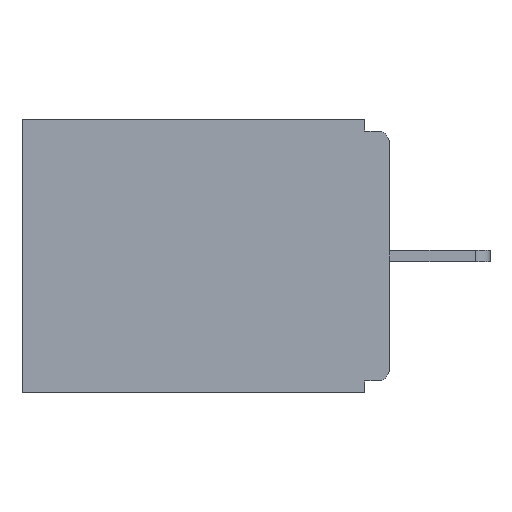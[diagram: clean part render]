
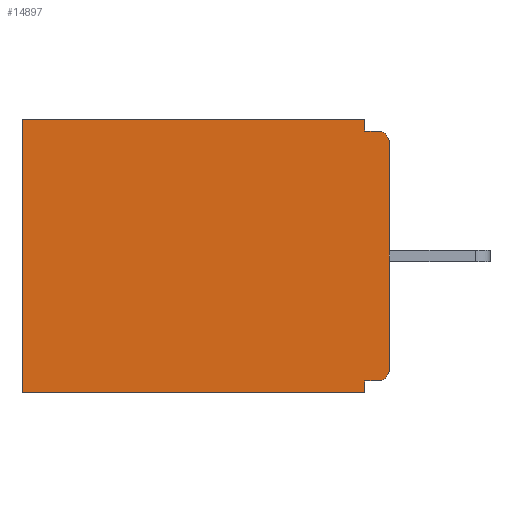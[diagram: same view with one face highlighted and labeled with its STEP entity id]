
A CAD part, left-side view. The second image highlights one B-rep face of the part: STEP entity #14897.
In plain terms, the highlighted planar face has unit normal (-1, 0, 0).
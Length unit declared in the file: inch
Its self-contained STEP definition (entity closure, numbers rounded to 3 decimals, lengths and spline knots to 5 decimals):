
#265 = EDGE_CURVE ( 'NONE', #14477, #7572, #15498, .T. ) ;
#371 = EDGE_CURVE ( 'NONE', #390, #12524, #1767, .T. ) ;
#390 = VERTEX_POINT ( 'NONE', #3162 ) ;
#401 = DIRECTION ( 'NONE',  ( 0., 1., 0. ) ) ;
#424 = CARTESIAN_POINT ( 'NONE',  ( 0.298, 0.031, -0.343 ) ) ;
#510 = DIRECTION ( 'NONE',  ( 0., 0., -1. ) ) ;
#1000 = ORIENTED_EDGE ( 'NONE', *, *, #10080, .T. ) ;
#1249 = VERTEX_POINT ( 'NONE', #15318 ) ;
#1595 = CARTESIAN_POINT ( 'NONE',  ( 0.298, 0.015, -0.015 ) ) ;
#1767 = CIRCLE ( 'NONE', #13955, 0.015 ) ;
#1855 = ORIENTED_EDGE ( 'NONE', *, *, #13545, .T. ) ;
#1878 = DIRECTION ( 'NONE',  ( -1., 0., 0. ) ) ;
#1902 = CARTESIAN_POINT ( 'NONE',  ( 0.298, 0.015, -0.313 ) ) ;
#2072 = DIRECTION ( 'NONE',  ( 0., -1., 0. ) ) ;
#2121 = EDGE_CURVE ( 'NONE', #4747, #12524, #15303, .T. ) ;
#2176 = CARTESIAN_POINT ( 'NONE',  ( 0.298, 0., -0.343 ) ) ;
#2389 = PLANE ( 'NONE',  #13708 ) ;
#2794 = DIRECTION ( 'NONE',  ( 0., 0., -1. ) ) ;
#2923 = FACE_OUTER_BOUND ( 'NONE', #7731, .T. ) ;
#3092 = EDGE_CURVE ( 'NONE', #7572, #6786, #9035, .T. ) ;
#3162 = CARTESIAN_POINT ( 'NONE',  ( 0.298, 0.015, -0.328 ) ) ;
#3292 = DIRECTION ( 'NONE',  ( 0., 0., -1. ) ) ;
#3473 = LINE ( 'NONE', #13514, #15269 ) ;
#3671 = DIRECTION ( 'NONE',  ( 0., 0., -1. ) ) ;
#4025 = ORIENTED_EDGE ( 'NONE', *, *, #11641, .F. ) ;
#4433 = ORIENTED_EDGE ( 'NONE', *, *, #13914, .T. ) ;
#4747 = VERTEX_POINT ( 'NONE', #12264 ) ;
#4798 = ORIENTED_EDGE ( 'NONE', *, *, #265, .F. ) ;
#5323 = VECTOR ( 'NONE', #15557, 39.37008 ) ;
#5744 = CIRCLE ( 'NONE', #6519, 0.015 ) ;
#5951 = VERTEX_POINT ( 'NONE', #9161 ) ;
#6136 = CARTESIAN_POINT ( 'NONE',  ( 0.298, 0., 0. ) ) ;
#6239 = VERTEX_POINT ( 'NONE', #12287 ) ;
#6481 = LINE ( 'NONE', #13273, #7225 ) ;
#6489 = CARTESIAN_POINT ( 'NONE',  ( 0.298, 0.031, 0. ) ) ;
#6519 = AXIS2_PLACEMENT_3D ( 'NONE', #13841, #6824, #14924 ) ;
#6579 = EDGE_CURVE ( 'NONE', #390, #1249, #6481, .T. ) ;
#6786 = VERTEX_POINT ( 'NONE', #1595 ) ;
#6824 = DIRECTION ( 'NONE',  ( -1., 0., 0. ) ) ;
#7225 = VECTOR ( 'NONE', #8311, 39.37008 ) ;
#7572 = VERTEX_POINT ( 'NONE', #7694 ) ;
#7694 = CARTESIAN_POINT ( 'NONE',  ( 0.298, 0.031, -0.015 ) ) ;
#7731 = EDGE_LOOP ( 'NONE', ( #1855, #13896, #4798, #1000, #4433, #10118, #4025, #14585, #8482, #14934 ) ) ;
#7816 = EDGE_CURVE ( 'NONE', #10622, #6239, #14106, .T. ) ;
#7980 = VECTOR ( 'NONE', #9443, 39.37008 ) ;
#8311 = DIRECTION ( 'NONE',  ( 0., 1., 0. ) ) ;
#8482 = ORIENTED_EDGE ( 'NONE', *, *, #371, .T. ) ;
#8664 = VECTOR ( 'NONE', #2072, 39.37008 ) ;
#8767 = CARTESIAN_POINT ( 'NONE',  ( 0.298, 0.46, 0. ) ) ;
#8950 = LINE ( 'NONE', #8767, #5323 ) ;
#9035 = LINE ( 'NONE', #9252, #8664 ) ;
#9161 = CARTESIAN_POINT ( 'NONE',  ( 0.298, 0.46, 0. ) ) ;
#9252 = CARTESIAN_POINT ( 'NONE',  ( 0.298, 0., -0.015 ) ) ;
#9385 = LINE ( 'NONE', #11911, #15061 ) ;
#9443 = DIRECTION ( 'NONE',  ( 0., 1., 0. ) ) ;
#10066 = CARTESIAN_POINT ( 'NONE',  ( 0.298, 0., -0.313 ) ) ;
#10080 = EDGE_CURVE ( 'NONE', #14477, #5951, #3473, .T. ) ;
#10118 = ORIENTED_EDGE ( 'NONE', *, *, #7816, .F. ) ;
#10256 = CARTESIAN_POINT ( 'NONE',  ( 0.298, 0., 0. ) ) ;
#10583 = VECTOR ( 'NONE', #510, 39.37008 ) ;
#10622 = VERTEX_POINT ( 'NONE', #13288 ) ;
#10917 = DIRECTION ( 'NONE',  ( 1., 0., 0. ) ) ;
#11641 = EDGE_CURVE ( 'NONE', #1249, #10622, #9385, .T. ) ;
#11911 = CARTESIAN_POINT ( 'NONE',  ( 0.298, 0.031, -0.343 ) ) ;
#12264 = CARTESIAN_POINT ( 'NONE',  ( 0.298, 0., -0.03 ) ) ;
#12287 = CARTESIAN_POINT ( 'NONE',  ( 0.298, 0.46, -0.343 ) ) ;
#12409 = VECTOR ( 'NONE', #3292, 39.37008 ) ;
#12524 = VERTEX_POINT ( 'NONE', #10066 ) ;
#13110 = DIRECTION ( 'NONE',  ( 0., 0., -1. ) ) ;
#13273 = CARTESIAN_POINT ( 'NONE',  ( 0.298, 0., -0.328 ) ) ;
#13288 = CARTESIAN_POINT ( 'NONE',  ( 0.298, 0.031, -0.343 ) ) ;
#13514 = CARTESIAN_POINT ( 'NONE',  ( 0.298, 0., 0. ) ) ;
#13545 = EDGE_CURVE ( 'NONE', #4747, #6786, #5744, .T. ) ;
#13708 = AXIS2_PLACEMENT_3D ( 'NONE', #6136, #10917, #3671 ) ;
#13841 = CARTESIAN_POINT ( 'NONE',  ( 0.298, 0.015, -0.03 ) ) ;
#13896 = ORIENTED_EDGE ( 'NONE', *, *, #3092, .F. ) ;
#13914 = EDGE_CURVE ( 'NONE', #5951, #6239, #8950, .T. ) ;
#13955 = AXIS2_PLACEMENT_3D ( 'NONE', #1902, #1878, #2794 ) ;
#14106 = LINE ( 'NONE', #2176, #7980 ) ;
#14477 = VERTEX_POINT ( 'NONE', #6489 ) ;
#14585 = ORIENTED_EDGE ( 'NONE', *, *, #6579, .F. ) ;
#14897 = ADVANCED_FACE ( 'NONE', ( #2923 ), #2389, .F. ) ;
#14924 = DIRECTION ( 'NONE',  ( 0., 0., -1. ) ) ;
#14934 = ORIENTED_EDGE ( 'NONE', *, *, #2121, .F. ) ;
#15061 = VECTOR ( 'NONE', #13110, 39.37008 ) ;
#15269 = VECTOR ( 'NONE', #401, 39.37008 ) ;
#15303 = LINE ( 'NONE', #10256, #12409 ) ;
#15318 = CARTESIAN_POINT ( 'NONE',  ( 0.298, 0.031, -0.328 ) ) ;
#15498 = LINE ( 'NONE', #424, #10583 ) ;
#15557 = DIRECTION ( 'NONE',  ( 0., 0., -1. ) ) ;
